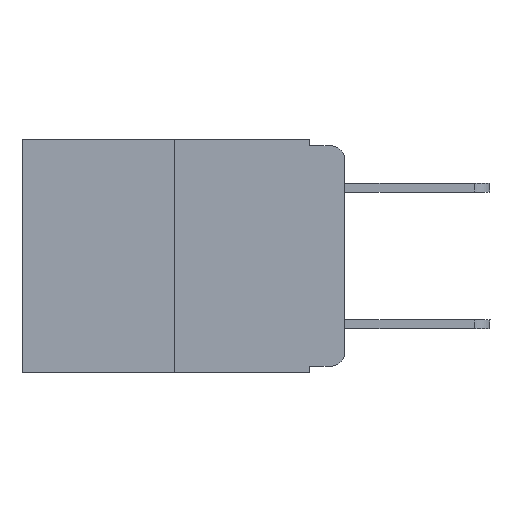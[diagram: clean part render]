
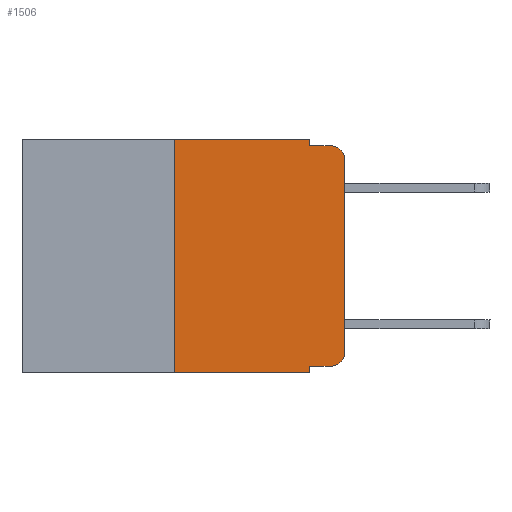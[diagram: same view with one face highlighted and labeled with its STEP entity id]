
A CAD part, left-side view. The second image highlights one B-rep face of the part: STEP entity #1506.
In plain terms, the highlighted planar face has unit normal (-1, 0, 0).
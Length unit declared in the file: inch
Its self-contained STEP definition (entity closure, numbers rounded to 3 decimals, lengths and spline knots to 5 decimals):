
#27 = CARTESIAN_POINT ( 'NONE',  ( 0., 0.473, 0. ) ) ;
#152 = LINE ( 'NONE', #7832, #4284 ) ;
#210 = CARTESIAN_POINT ( 'NONE',  ( 0., 0.25, 0. ) ) ;
#219 = DIRECTION ( 'NONE',  ( 0., 0., 1. ) ) ;
#385 = VERTEX_POINT ( 'NONE', #210 ) ;
#562 = CIRCLE ( 'NONE', #3787, 0.02 ) ;
#672 = VECTOR ( 'NONE', #2954, 39.37008 ) ;
#755 = CARTESIAN_POINT ( 'NONE',  ( 0., 0.02, -0.01 ) ) ;
#858 = CARTESIAN_POINT ( 'NONE',  ( 0., 0.051, -0.333 ) ) ;
#890 = CARTESIAN_POINT ( 'NONE',  ( 0., 0.051, -0.01 ) ) ;
#908 = VERTEX_POINT ( 'NONE', #4108 ) ;
#1291 = CARTESIAN_POINT ( 'NONE',  ( 0., 0.02, -0.03 ) ) ;
#1361 = CARTESIAN_POINT ( 'NONE',  ( 0., 0.051, -0.333 ) ) ;
#1506 = ADVANCED_FACE ( 'NONE', ( #7337 ), #3374, .F. ) ;
#1815 = EDGE_CURVE ( 'NONE', #7221, #5467, #152, .T. ) ;
#1818 = EDGE_CURVE ( 'NONE', #7221, #385, #5836, .T. ) ;
#2201 = LINE ( 'NONE', #10963, #4355 ) ;
#2232 = DIRECTION ( 'NONE',  ( 0., 0., -1. ) ) ;
#2631 = ORIENTED_EDGE ( 'NONE', *, *, #3897, .F. ) ;
#2682 = CARTESIAN_POINT ( 'NONE',  ( 0., 0., -0.313 ) ) ;
#2808 = LINE ( 'NONE', #6653, #5195 ) ;
#2812 = LINE ( 'NONE', #858, #7729 ) ;
#2954 = DIRECTION ( 'NONE',  ( 0., 0., -1. ) ) ;
#3193 = CARTESIAN_POINT ( 'NONE',  ( 0., 0.02, -0.313 ) ) ;
#3374 = PLANE ( 'NONE',  #7825 ) ;
#3517 = CARTESIAN_POINT ( 'NONE',  ( 0., 0., 0. ) ) ;
#3577 = LINE ( 'NONE', #3517, #3778 ) ;
#3620 = ORIENTED_EDGE ( 'NONE', *, *, #11925, .T. ) ;
#3716 = ORIENTED_EDGE ( 'NONE', *, *, #4138, .F. ) ;
#3778 = VECTOR ( 'NONE', #4542, 39.37008 ) ;
#3787 = AXIS2_PLACEMENT_3D ( 'NONE', #1291, #9003, #2232 ) ;
#3897 = EDGE_CURVE ( 'NONE', #5218, #5467, #11973, .T. ) ;
#3988 = CARTESIAN_POINT ( 'NONE',  ( 0., 0., -0.03 ) ) ;
#4099 = VECTOR ( 'NONE', #219, 39.37008 ) ;
#4108 = CARTESIAN_POINT ( 'NONE',  ( 0., 0.02, -0.333 ) ) ;
#4138 = EDGE_CURVE ( 'NONE', #6549, #7687, #2808, .T. ) ;
#4284 = VECTOR ( 'NONE', #5950, 39.37008 ) ;
#4355 = VECTOR ( 'NONE', #9028, 39.37008 ) ;
#4527 = DIRECTION ( 'NONE',  ( 1., 0., 0. ) ) ;
#4542 = DIRECTION ( 'NONE',  ( 0., 0., 1. ) ) ;
#4585 = VECTOR ( 'NONE', #4954, 39.37008 ) ;
#4769 = ORIENTED_EDGE ( 'NONE', *, *, #12069, .T. ) ;
#4954 = DIRECTION ( 'NONE',  ( 0., -1., 0. ) ) ;
#4987 = DIRECTION ( 'NONE',  ( -1., 0., 0. ) ) ;
#5195 = VECTOR ( 'NONE', #9576, 39.37008 ) ;
#5218 = VERTEX_POINT ( 'NONE', #1361 ) ;
#5399 = CARTESIAN_POINT ( 'NONE',  ( 0., 0.051, 0. ) ) ;
#5467 = VERTEX_POINT ( 'NONE', #9513 ) ;
#5788 = CIRCLE ( 'NONE', #6381, 0.02 ) ;
#5836 = LINE ( 'NONE', #9811, #4099 ) ;
#5880 = ORIENTED_EDGE ( 'NONE', *, *, #10284, .F. ) ;
#5950 = DIRECTION ( 'NONE',  ( 0., -1., 0. ) ) ;
#5964 = EDGE_LOOP ( 'NONE', ( #4769, #6651, #5880, #3716, #8965, #6952, #8300, #2631, #10825, #3620 ) ) ;
#5979 = DIRECTION ( 'NONE',  ( 0., 0., -1. ) ) ;
#6381 = AXIS2_PLACEMENT_3D ( 'NONE', #3193, #4987, #5979 ) ;
#6549 = VERTEX_POINT ( 'NONE', #5399 ) ;
#6651 = ORIENTED_EDGE ( 'NONE', *, *, #12456, .T. ) ;
#6653 = CARTESIAN_POINT ( 'NONE',  ( 0., 0.051, 0. ) ) ;
#6952 = ORIENTED_EDGE ( 'NONE', *, *, #1818, .F. ) ;
#7209 = CARTESIAN_POINT ( 'NONE',  ( 0., 0.473, 0. ) ) ;
#7221 = VERTEX_POINT ( 'NONE', #10563 ) ;
#7337 = FACE_OUTER_BOUND ( 'NONE', #5964, .T. ) ;
#7687 = VERTEX_POINT ( 'NONE', #890 ) ;
#7729 = VECTOR ( 'NONE', #9578, 39.37008 ) ;
#7825 = AXIS2_PLACEMENT_3D ( 'NONE', #7209, #4527, #11077 ) ;
#7832 = CARTESIAN_POINT ( 'NONE',  ( 0., 0.473, -0.343 ) ) ;
#8300 = ORIENTED_EDGE ( 'NONE', *, *, #1815, .T. ) ;
#8952 = VERTEX_POINT ( 'NONE', #3988 ) ;
#8965 = ORIENTED_EDGE ( 'NONE', *, *, #11608, .F. ) ;
#9003 = DIRECTION ( 'NONE',  ( -1., 0., 0. ) ) ;
#9028 = DIRECTION ( 'NONE',  ( 0., -1., 0. ) ) ;
#9513 = CARTESIAN_POINT ( 'NONE',  ( 0., 0.051, -0.343 ) ) ;
#9576 = DIRECTION ( 'NONE',  ( 0., 0., -1. ) ) ;
#9578 = DIRECTION ( 'NONE',  ( 0., -1., 0. ) ) ;
#9660 = EDGE_CURVE ( 'NONE', #5218, #908, #2812, .T. ) ;
#9799 = VERTEX_POINT ( 'NONE', #2682 ) ;
#9811 = CARTESIAN_POINT ( 'NONE',  ( 0., 0.25, 0. ) ) ;
#10284 = EDGE_CURVE ( 'NONE', #7687, #10561, #2201, .T. ) ;
#10561 = VERTEX_POINT ( 'NONE', #755 ) ;
#10563 = CARTESIAN_POINT ( 'NONE',  ( 0., 0.25, -0.343 ) ) ;
#10742 = LINE ( 'NONE', #27, #4585 ) ;
#10787 = CARTESIAN_POINT ( 'NONE',  ( 0., 0.051, 0. ) ) ;
#10825 = ORIENTED_EDGE ( 'NONE', *, *, #9660, .T. ) ;
#10963 = CARTESIAN_POINT ( 'NONE',  ( 0., 0.051, -0.01 ) ) ;
#11077 = DIRECTION ( 'NONE',  ( 0., 0., -1. ) ) ;
#11608 = EDGE_CURVE ( 'NONE', #385, #6549, #10742, .T. ) ;
#11925 = EDGE_CURVE ( 'NONE', #908, #9799, #5788, .T. ) ;
#11973 = LINE ( 'NONE', #10787, #672 ) ;
#12069 = EDGE_CURVE ( 'NONE', #9799, #8952, #3577, .T. ) ;
#12456 = EDGE_CURVE ( 'NONE', #8952, #10561, #562, .T. ) ;
